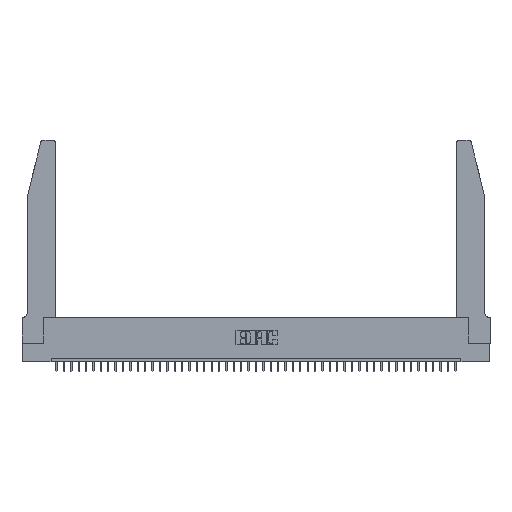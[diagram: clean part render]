
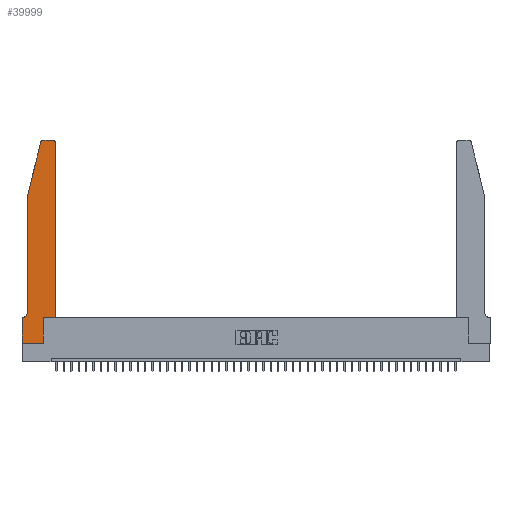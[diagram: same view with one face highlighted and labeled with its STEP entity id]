
A CAD part, top view. The second image highlights one B-rep face of the part: STEP entity #39999.
In plain terms, the highlighted planar face has unit normal (0, 0, 1).
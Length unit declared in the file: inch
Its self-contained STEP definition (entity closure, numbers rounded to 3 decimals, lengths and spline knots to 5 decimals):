
#262 = VERTEX_POINT ( 'NONE', #1566 ) ;
#460 = CARTESIAN_POINT ( 'NONE',  ( 0.4205, 2.72, 0.37 ) ) ;
#1268 = VERTEX_POINT ( 'NONE', #40964 ) ;
#1330 = CARTESIAN_POINT ( 'NONE',  ( 0.2865, 0.35, 0.37 ) ) ;
#1351 = CARTESIAN_POINT ( 'NONE',  ( 0.0755, 2., 0.37 ) ) ;
#1409 = CARTESIAN_POINT ( 'NONE',  ( 0.0755, 0.42, 0.37 ) ) ;
#1495 = ORIENTED_EDGE ( 'NONE', *, *, #8123, .T. ) ;
#1566 = CARTESIAN_POINT ( 'NONE',  ( 0., 0., 0.37 ) ) ;
#1604 = EDGE_CURVE ( 'NONE', #28803, #40834, #43184, .T. ) ;
#2597 = DIRECTION ( 'NONE',  ( 0., 0., -1. ) ) ;
#2663 = VERTEX_POINT ( 'NONE', #1409 ) ;
#4001 = AXIS2_PLACEMENT_3D ( 'NONE', #12914, #36539, #5729 ) ;
#4283 = DIRECTION ( 'NONE',  ( 0., 0., 1. ) ) ;
#4555 = EDGE_CURVE ( 'NONE', #36277, #2663, #4714, .T. ) ;
#4714 = LINE ( 'NONE', #1351, #9068 ) ;
#4900 = DIRECTION ( 'NONE',  ( 0., 0., 1. ) ) ;
#5179 = CARTESIAN_POINT ( 'NONE',  ( 0., 0.35, 0.37 ) ) ;
#5729 = DIRECTION ( 'NONE',  ( 1., 0., 0. ) ) ;
#6254 = VECTOR ( 'NONE', #28322, 39.37008 ) ;
#6981 = CARTESIAN_POINT ( 'NONE',  ( 0., 0., 0.37 ) ) ;
#7193 = ORIENTED_EDGE ( 'NONE', *, *, #1604, .T. ) ;
#7425 = CARTESIAN_POINT ( 'NONE',  ( 0.0055, 0.35, 0.37 ) ) ;
#7656 = EDGE_CURVE ( 'NONE', #29053, #1268, #21120, .T. ) ;
#7729 = ORIENTED_EDGE ( 'NONE', *, *, #12526, .T. ) ;
#8123 = EDGE_CURVE ( 'NONE', #37386, #22281, #10935, .T. ) ;
#8127 = ORIENTED_EDGE ( 'NONE', *, *, #30636, .T. ) ;
#8805 = CARTESIAN_POINT ( 'NONE',  ( 0.284, 2.75, 0.37 ) ) ;
#8970 = DIRECTION ( 'NONE',  ( -1., 0., 0. ) ) ;
#9068 = VECTOR ( 'NONE', #32392, 39.37008 ) ;
#9611 = EDGE_LOOP ( 'NONE', ( #1495, #8127, #38480, #40140, #21882, #7193, #23232, #24110, #22327, #44156, #7729, #11808 ) ) ;
#9669 = VERTEX_POINT ( 'NONE', #16328 ) ;
#10935 = LINE ( 'NONE', #24675, #32291 ) ;
#11808 = ORIENTED_EDGE ( 'NONE', *, *, #41934, .T. ) ;
#12526 = EDGE_CURVE ( 'NONE', #9669, #30009, #12868, .T. ) ;
#12868 = LINE ( 'NONE', #26575, #13751 ) ;
#12914 = CARTESIAN_POINT ( 'NONE',  ( 0., 0.35, 0.37 ) ) ;
#13751 = VECTOR ( 'NONE', #36930, 39.37008 ) ;
#13911 = VERTEX_POINT ( 'NONE', #27912 ) ;
#14385 = LINE ( 'NONE', #34844, #6254 ) ;
#15060 = DIRECTION ( 'NONE',  ( 0., 1., 0. ) ) ;
#16328 = CARTESIAN_POINT ( 'NONE',  ( 0.4505, 0.35, 0.37 ) ) ;
#16393 = CIRCLE ( 'NONE', #22144, 0.07 ) ;
#17266 = CARTESIAN_POINT ( 'NONE',  ( 0.0755, 2., 0.37 ) ) ;
#17321 = EDGE_CURVE ( 'NONE', #13911, #36277, #38400, .T. ) ;
#17995 = DIRECTION ( 'NONE',  ( 1., 0., 0. ) ) ;
#18226 = EDGE_CURVE ( 'NONE', #40834, #262, #38244, .T. ) ;
#18620 = DIRECTION ( 'NONE',  ( 1., 0., 0. ) ) ;
#19679 = VECTOR ( 'NONE', #30990, 39.37008 ) ;
#20492 = CARTESIAN_POINT ( 'NONE',  ( 0.4505, 2.72, 0.37 ) ) ;
#21120 = LINE ( 'NONE', #1330, #27914 ) ;
#21285 = DIRECTION ( 'NONE',  ( -1., 0., 0. ) ) ;
#21366 = DIRECTION ( 'NONE',  ( 0., -1., 0. ) ) ;
#21882 = ORIENTED_EDGE ( 'NONE', *, *, #43632, .T. ) ;
#22144 = AXIS2_PLACEMENT_3D ( 'NONE', #23492, #2597, #37217 ) ;
#22281 = VERTEX_POINT ( 'NONE', #8805 ) ;
#22327 = ORIENTED_EDGE ( 'NONE', *, *, #7656, .T. ) ;
#22569 = EDGE_CURVE ( 'NONE', #262, #29053, #14385, .T. ) ;
#22917 = LINE ( 'NONE', #32835, #30389 ) ;
#23146 = VECTOR ( 'NONE', #8970, 39.37008 ) ;
#23232 = ORIENTED_EDGE ( 'NONE', *, *, #18226, .T. ) ;
#23492 = CARTESIAN_POINT ( 'NONE',  ( 0.0055, 0.42, 0.37 ) ) ;
#24110 = ORIENTED_EDGE ( 'NONE', *, *, #22569, .T. ) ;
#24675 = CARTESIAN_POINT ( 'NONE',  ( 0.2605, 2.75, 0.37 ) ) ;
#26071 = CARTESIAN_POINT ( 'NONE',  ( 0.0755, 0.35, 0.37 ) ) ;
#26189 = FACE_OUTER_BOUND ( 'NONE', #9611, .T. ) ;
#26295 = CARTESIAN_POINT ( 'NONE',  ( 0.2865, 0., 0.37 ) ) ;
#26575 = CARTESIAN_POINT ( 'NONE',  ( 0.4505, 0.35, 0.37 ) ) ;
#27912 = CARTESIAN_POINT ( 'NONE',  ( 0.25487, 2.72718, 0.37 ) ) ;
#27914 = VECTOR ( 'NONE', #15060, 39.37008 ) ;
#28201 = CIRCLE ( 'NONE', #28946, 0.03 ) ;
#28322 = DIRECTION ( 'NONE',  ( 1., 0., 0. ) ) ;
#28803 = VERTEX_POINT ( 'NONE', #7425 ) ;
#28946 = AXIS2_PLACEMENT_3D ( 'NONE', #35716, #4900, #18620 ) ;
#29053 = VERTEX_POINT ( 'NONE', #26295 ) ;
#30009 = VERTEX_POINT ( 'NONE', #20492 ) ;
#30389 = VECTOR ( 'NONE', #36642, 39.37008 ) ;
#30636 = EDGE_CURVE ( 'NONE', #22281, #13911, #28201, .T. ) ;
#30990 = DIRECTION ( 'NONE',  ( -0.239, -0.971, 0. ) ) ;
#32050 = CARTESIAN_POINT ( 'NONE',  ( 0.4205, 2.75, 0.37 ) ) ;
#32291 = VECTOR ( 'NONE', #21285, 39.37008 ) ;
#32392 = DIRECTION ( 'NONE',  ( 0., -1., 0. ) ) ;
#32835 = CARTESIAN_POINT ( 'NONE',  ( 0.4505, 0.35, 0.37 ) ) ;
#34844 = CARTESIAN_POINT ( 'NONE',  ( 0., 0., 0.37 ) ) ;
#35716 = CARTESIAN_POINT ( 'NONE',  ( 0.284, 2.72, 0.37 ) ) ;
#36277 = VERTEX_POINT ( 'NONE', #43018 ) ;
#36287 = VECTOR ( 'NONE', #21366, 39.37008 ) ;
#36320 = PLANE ( 'NONE',  #4001 ) ;
#36468 = AXIS2_PLACEMENT_3D ( 'NONE', #460, #4283, #17995 ) ;
#36539 = DIRECTION ( 'NONE',  ( 0., 0., 1. ) ) ;
#36564 = EDGE_CURVE ( 'NONE', #1268, #9669, #22917, .T. ) ;
#36642 = DIRECTION ( 'NONE',  ( 1., 0., 0. ) ) ;
#36930 = DIRECTION ( 'NONE',  ( 0., 1., 0. ) ) ;
#37217 = DIRECTION ( 'NONE',  ( -1., 0., 0. ) ) ;
#37386 = VERTEX_POINT ( 'NONE', #32050 ) ;
#38244 = LINE ( 'NONE', #6981, #36287 ) ;
#38400 = LINE ( 'NONE', #17266, #19679 ) ;
#38480 = ORIENTED_EDGE ( 'NONE', *, *, #17321, .T. ) ;
#39999 = ADVANCED_FACE ( 'NONE', ( #26189 ), #36320, .T. ) ;
#40140 = ORIENTED_EDGE ( 'NONE', *, *, #4555, .T. ) ;
#40778 = CIRCLE ( 'NONE', #36468, 0.03 ) ;
#40834 = VERTEX_POINT ( 'NONE', #5179 ) ;
#40964 = CARTESIAN_POINT ( 'NONE',  ( 0.2865, 0.35, 0.37 ) ) ;
#41934 = EDGE_CURVE ( 'NONE', #30009, #37386, #40778, .T. ) ;
#43018 = CARTESIAN_POINT ( 'NONE',  ( 0.0755, 2., 0.37 ) ) ;
#43184 = LINE ( 'NONE', #26071, #23146 ) ;
#43632 = EDGE_CURVE ( 'NONE', #2663, #28803, #16393, .T. ) ;
#44156 = ORIENTED_EDGE ( 'NONE', *, *, #36564, .T. ) ;
